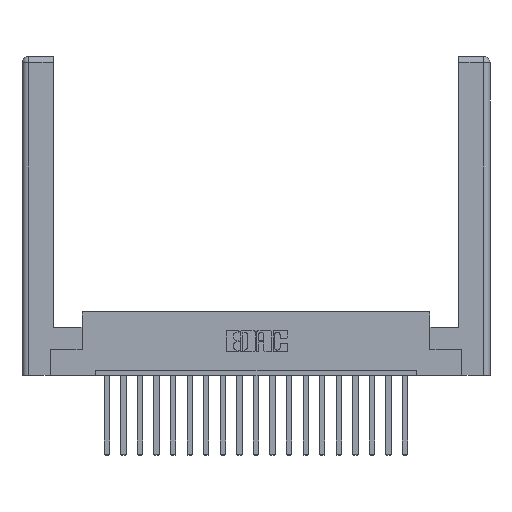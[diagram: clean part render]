
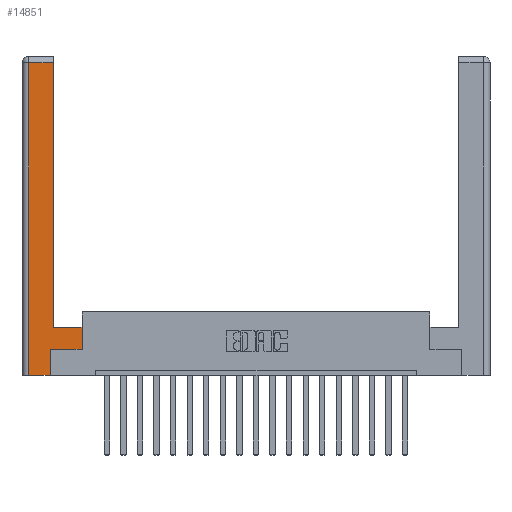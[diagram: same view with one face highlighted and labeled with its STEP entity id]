
A CAD part, top view. The second image highlights one B-rep face of the part: STEP entity #14851.
In plain terms, the highlighted planar face has unit normal (0, 0, 1).
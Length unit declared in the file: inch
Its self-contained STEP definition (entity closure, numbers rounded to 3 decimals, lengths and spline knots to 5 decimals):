
#216 = FACE_OUTER_BOUND ( 'NONE', #16817, .T. ) ;
#272 = LINE ( 'NONE', #8009, #3838 ) ;
#827 = CARTESIAN_POINT ( 'NONE',  ( 0.295, 3., 0. ) ) ;
#830 = DIRECTION ( 'NONE',  ( 0., -1., 0. ) ) ;
#1339 = VECTOR ( 'NONE', #16050, 39.37008 ) ;
#1347 = CARTESIAN_POINT ( 'NONE',  ( 0.565, 0.45, 0. ) ) ;
#1498 = VECTOR ( 'NONE', #17488, 39.37008 ) ;
#1509 = DIRECTION ( 'NONE',  ( 1., 0., 0. ) ) ;
#1601 = CARTESIAN_POINT ( 'NONE',  ( 0.0615, 2.94, 0. ) ) ;
#1734 = AXIS2_PLACEMENT_3D ( 'NONE', #11737, #16197, #13276 ) ;
#2647 = VERTEX_POINT ( 'NONE', #6952 ) ;
#2794 = VERTEX_POINT ( 'NONE', #14992 ) ;
#2827 = CARTESIAN_POINT ( 'NONE',  ( 0.295, 0.45, 0. ) ) ;
#3276 = DIRECTION ( 'NONE',  ( 0., 1., 0. ) ) ;
#3352 = ORIENTED_EDGE ( 'NONE', *, *, #10289, .T. ) ;
#3456 = LINE ( 'NONE', #16390, #18571 ) ;
#3569 = ORIENTED_EDGE ( 'NONE', *, *, #5974, .T. ) ;
#3838 = VECTOR ( 'NONE', #3276, 39.37008 ) ;
#3888 = ORIENTED_EDGE ( 'NONE', *, *, #6625, .T. ) ;
#5052 = ORIENTED_EDGE ( 'NONE', *, *, #15315, .T. ) ;
#5110 = EDGE_CURVE ( 'NONE', #7756, #12043, #3456, .T. ) ;
#5254 = ORIENTED_EDGE ( 'NONE', *, *, #12481, .T. ) ;
#5974 = EDGE_CURVE ( 'NONE', #7666, #12971, #8137, .T. ) ;
#6411 = VERTEX_POINT ( 'NONE', #6836 ) ;
#6580 = CARTESIAN_POINT ( 'NONE',  ( 0.565, 0.245, 0. ) ) ;
#6625 = EDGE_CURVE ( 'NONE', #17455, #2794, #16870, .T. ) ;
#6836 = CARTESIAN_POINT ( 'NONE',  ( 0.265, 0., 0. ) ) ;
#6952 = CARTESIAN_POINT ( 'NONE',  ( 0.0615, 0., 0. ) ) ;
#7666 = VERTEX_POINT ( 'NONE', #13304 ) ;
#7726 = LINE ( 'NONE', #1347, #9359 ) ;
#7756 = VERTEX_POINT ( 'NONE', #11345 ) ;
#8009 = CARTESIAN_POINT ( 'NONE',  ( 0.265, 0.245, 0. ) ) ;
#8137 = LINE ( 'NONE', #14587, #1498 ) ;
#8455 = VECTOR ( 'NONE', #830, 39.37008 ) ;
#9182 = CARTESIAN_POINT ( 'NONE',  ( 0.0615, 0., 0. ) ) ;
#9359 = VECTOR ( 'NONE', #19376, 39.37008 ) ;
#10004 = EDGE_CURVE ( 'NONE', #12043, #17455, #19525, .T. ) ;
#10205 = PLANE ( 'NONE',  #1734 ) ;
#10289 = EDGE_CURVE ( 'NONE', #12971, #7756, #7726, .T. ) ;
#10575 = CARTESIAN_POINT ( 'NONE',  ( 0.265, 0., 0. ) ) ;
#10792 = CARTESIAN_POINT ( 'NONE',  ( 0.295, 2.94, 0. ) ) ;
#11345 = CARTESIAN_POINT ( 'NONE',  ( 0.565, 0.45, 0. ) ) ;
#11737 = CARTESIAN_POINT ( 'NONE',  ( 0., 0., 0. ) ) ;
#12033 = ORIENTED_EDGE ( 'NONE', *, *, #17475, .T. ) ;
#12043 = VERTEX_POINT ( 'NONE', #2827 ) ;
#12481 = EDGE_CURVE ( 'NONE', #2647, #6411, #14255, .T. ) ;
#12971 = VERTEX_POINT ( 'NONE', #6580 ) ;
#13187 = LINE ( 'NONE', #9182, #8455 ) ;
#13276 = DIRECTION ( 'NONE',  ( -1., 0., 0. ) ) ;
#13304 = CARTESIAN_POINT ( 'NONE',  ( 0.265, 0.245, 0. ) ) ;
#13790 = VECTOR ( 'NONE', #1509, 39.37008 ) ;
#13970 = DIRECTION ( 'NONE',  ( -1., 0., 0. ) ) ;
#14255 = LINE ( 'NONE', #10575, #13790 ) ;
#14552 = ORIENTED_EDGE ( 'NONE', *, *, #10004, .T. ) ;
#14587 = CARTESIAN_POINT ( 'NONE',  ( 0.565, 0.245, 0. ) ) ;
#14851 = ADVANCED_FACE ( 'NONE', ( #216 ), #10205, .F. ) ;
#14959 = VECTOR ( 'NONE', #13970, 39.37008 ) ;
#14992 = CARTESIAN_POINT ( 'NONE',  ( 0.0615, 2.94, 0. ) ) ;
#15315 = EDGE_CURVE ( 'NONE', #2794, #2647, #13187, .T. ) ;
#16050 = DIRECTION ( 'NONE',  ( 0., 1., 0. ) ) ;
#16162 = ORIENTED_EDGE ( 'NONE', *, *, #5110, .T. ) ;
#16197 = DIRECTION ( 'NONE',  ( 0., 0., -1. ) ) ;
#16257 = DIRECTION ( 'NONE',  ( -1., 0., 0. ) ) ;
#16390 = CARTESIAN_POINT ( 'NONE',  ( 0.295, 0.45, 0. ) ) ;
#16817 = EDGE_LOOP ( 'NONE', ( #14552, #3888, #5052, #5254, #12033, #3569, #3352, #16162 ) ) ;
#16870 = LINE ( 'NONE', #1601, #14959 ) ;
#17455 = VERTEX_POINT ( 'NONE', #10792 ) ;
#17475 = EDGE_CURVE ( 'NONE', #6411, #7666, #272, .T. ) ;
#17488 = DIRECTION ( 'NONE',  ( 1., 0., 0. ) ) ;
#18571 = VECTOR ( 'NONE', #16257, 39.37008 ) ;
#19376 = DIRECTION ( 'NONE',  ( 0., 1., 0. ) ) ;
#19525 = LINE ( 'NONE', #827, #1339 ) ;
